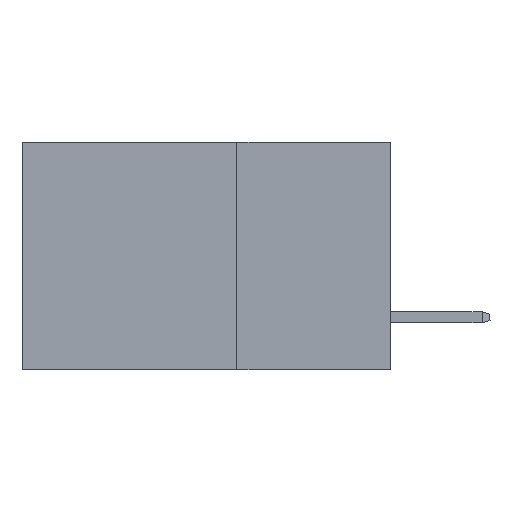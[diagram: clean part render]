
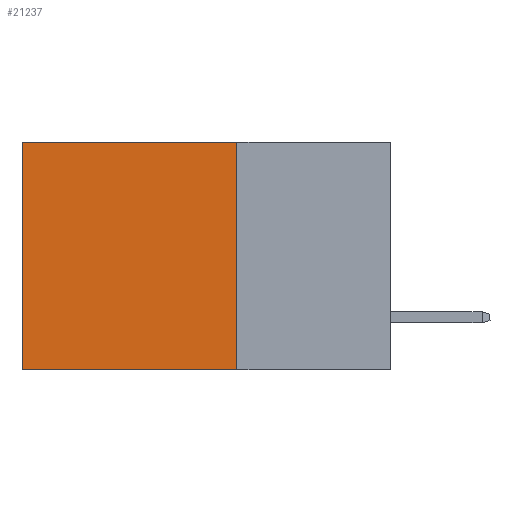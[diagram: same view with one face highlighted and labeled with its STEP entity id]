
A CAD part, left-side view. The second image highlights one B-rep face of the part: STEP entity #21237.
In plain terms, the highlighted planar face has unit normal (-1, 0, 0).
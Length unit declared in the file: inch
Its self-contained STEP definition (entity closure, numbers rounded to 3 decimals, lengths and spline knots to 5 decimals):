
#726 = CARTESIAN_POINT ( 'NONE',  ( 0.2875, 0.25, 0. ) ) ;
#1284 = EDGE_CURVE ( 'NONE', #17059, #12492, #7480, .T. ) ;
#1447 = DIRECTION ( 'NONE',  ( 0., 1., 0. ) ) ;
#2047 = AXIS2_PLACEMENT_3D ( 'NONE', #726, #15623, #2919 ) ;
#2624 = EDGE_CURVE ( 'NONE', #25791, #17059, #25017, .T. ) ;
#2919 = DIRECTION ( 'NONE',  ( 0., 0., -1. ) ) ;
#3080 = EDGE_LOOP ( 'NONE', ( #16227, #24753, #4508, #17523 ) ) ;
#4095 = FACE_OUTER_BOUND ( 'NONE', #3080, .T. ) ;
#4508 = ORIENTED_EDGE ( 'NONE', *, *, #12462, .F. ) ;
#6540 = DIRECTION ( 'NONE',  ( 0., 0., -1. ) ) ;
#6629 = VERTEX_POINT ( 'NONE', #17738 ) ;
#6636 = CARTESIAN_POINT ( 'NONE',  ( 0.2875, 0.6, -0.37 ) ) ;
#7001 = DIRECTION ( 'NONE',  ( 0., 1., 0. ) ) ;
#7480 = LINE ( 'NONE', #18892, #18640 ) ;
#9379 = VECTOR ( 'NONE', #6540, 39.37008 ) ;
#10052 = LINE ( 'NONE', #12834, #9379 ) ;
#12462 = EDGE_CURVE ( 'NONE', #25791, #6629, #10052, .T. ) ;
#12492 = VERTEX_POINT ( 'NONE', #6636 ) ;
#12834 = CARTESIAN_POINT ( 'NONE',  ( 0.2875, 0.25, 0. ) ) ;
#13982 = VECTOR ( 'NONE', #7001, 39.37008 ) ;
#13989 = CARTESIAN_POINT ( 'NONE',  ( 0.2875, 0.25, 0. ) ) ;
#14340 = CARTESIAN_POINT ( 'NONE',  ( 0.2875, 0.6, 0. ) ) ;
#15399 = VECTOR ( 'NONE', #1447, 39.37008 ) ;
#15623 = DIRECTION ( 'NONE',  ( 1., 0., 0. ) ) ;
#16227 = ORIENTED_EDGE ( 'NONE', *, *, #1284, .T. ) ;
#17059 = VERTEX_POINT ( 'NONE', #14340 ) ;
#17523 = ORIENTED_EDGE ( 'NONE', *, *, #2624, .T. ) ;
#17738 = CARTESIAN_POINT ( 'NONE',  ( 0.2875, 0.25, -0.37 ) ) ;
#18640 = VECTOR ( 'NONE', #26881, 39.37008 ) ;
#18892 = CARTESIAN_POINT ( 'NONE',  ( 0.2875, 0.6, 0. ) ) ;
#20792 = EDGE_CURVE ( 'NONE', #6629, #12492, #20944, .T. ) ;
#20944 = LINE ( 'NONE', #22473, #15399 ) ;
#21237 = ADVANCED_FACE ( 'NONE', ( #4095 ), #21822, .F. ) ;
#21822 = PLANE ( 'NONE',  #2047 ) ;
#22473 = CARTESIAN_POINT ( 'NONE',  ( 0.2875, 0.25, -0.37 ) ) ;
#24753 = ORIENTED_EDGE ( 'NONE', *, *, #20792, .F. ) ;
#25017 = LINE ( 'NONE', #25789, #13982 ) ;
#25789 = CARTESIAN_POINT ( 'NONE',  ( 0.2875, 0.25, 0. ) ) ;
#25791 = VERTEX_POINT ( 'NONE', #13989 ) ;
#26881 = DIRECTION ( 'NONE',  ( 0., 0., -1. ) ) ;
